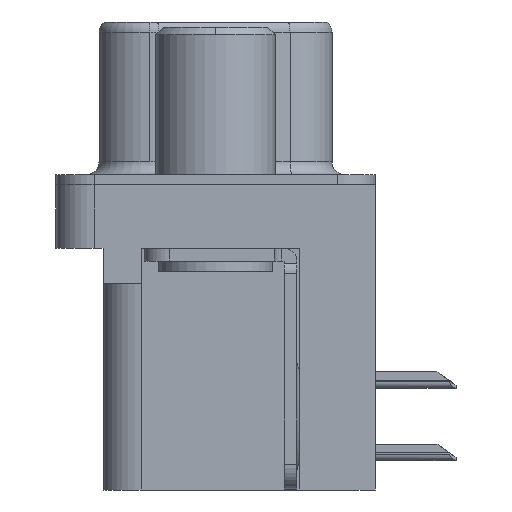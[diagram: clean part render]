
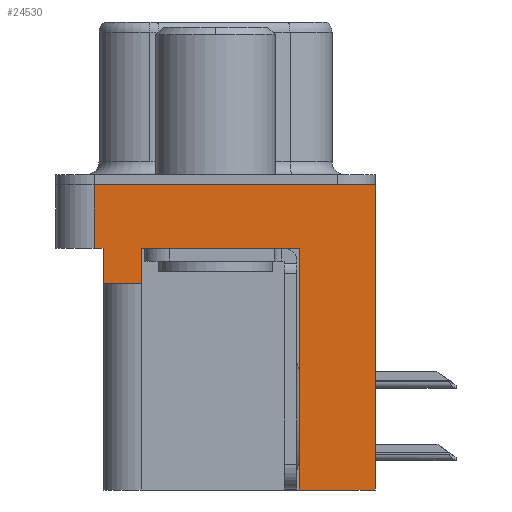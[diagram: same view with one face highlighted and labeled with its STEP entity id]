
A CAD part, left-side view. The second image highlights one B-rep face of the part: STEP entity #24530.
In plain terms, the highlighted planar face has unit normal (-1, 0, 0).
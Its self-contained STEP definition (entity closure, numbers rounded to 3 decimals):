
#223 = EDGE_CURVE ( 'NONE', #3522, #14569, #980, .T. ) ;
#358 = VECTOR ( 'NONE', #23700, 1000. ) ;
#980 = LINE ( 'NONE', #25428, #28120 ) ;
#1089 = EDGE_CURVE ( 'NONE', #8767, #10341, #22479, .T. ) ;
#1161 = CARTESIAN_POINT ( 'NONE',  ( -2.91, 2.895, -2.5 ) ) ;
#1478 = CARTESIAN_POINT ( 'NONE',  ( -2.91, -6.275, -2.5 ) ) ;
#2150 = VECTOR ( 'NONE', #5398, 1000. ) ;
#2228 = ORIENTED_EDGE ( 'NONE', *, *, #223, .T. ) ;
#2453 = CARTESIAN_POINT ( 'NONE',  ( -2.91, -6.275, -12. ) ) ;
#2769 = DIRECTION ( 'NONE',  ( 0., 0., 1. ) ) ;
#3426 = VERTEX_POINT ( 'NONE', #7520 ) ;
#3522 = VERTEX_POINT ( 'NONE', #1161 ) ;
#3541 = DIRECTION ( 'NONE',  ( 0., 0., 1. ) ) ;
#3948 = CARTESIAN_POINT ( 'NONE',  ( -2.91, 2.895, -3.9 ) ) ;
#4138 = ORIENTED_EDGE ( 'NONE', *, *, #10745, .F. ) ;
#4487 = EDGE_CURVE ( 'NONE', #10341, #17937, #27264, .T. ) ;
#4972 = LINE ( 'NONE', #16119, #2150 ) ;
#5138 = VECTOR ( 'NONE', #26257, 1000. ) ;
#5398 = DIRECTION ( 'NONE',  ( 0., 0., 1. ) ) ;
#5676 = ORIENTED_EDGE ( 'NONE', *, *, #19729, .F. ) ;
#5688 = VECTOR ( 'NONE', #17936, 1000. ) ;
#6105 = VECTOR ( 'NONE', #27433, 1000. ) ;
#6129 = CARTESIAN_POINT ( 'NONE',  ( -2.91, -3.295, -12. ) ) ;
#6491 = CARTESIAN_POINT ( 'NONE',  ( -2.91, -6.275, -2.5 ) ) ;
#6567 = ORIENTED_EDGE ( 'NONE', *, *, #21819, .F. ) ;
#6787 = DIRECTION ( 'NONE',  ( 0., -1., 0. ) ) ;
#7002 = LINE ( 'NONE', #1478, #358 ) ;
#7406 = LINE ( 'NONE', #27875, #10152 ) ;
#7520 = CARTESIAN_POINT ( 'NONE',  ( -2.91, 4.775, 0. ) ) ;
#8543 = EDGE_CURVE ( 'NONE', #8767, #3522, #23124, .T. ) ;
#8767 = VERTEX_POINT ( 'NONE', #3948 ) ;
#9052 = CARTESIAN_POINT ( 'NONE',  ( -2.91, -6.275, 0. ) ) ;
#9669 = DIRECTION ( 'NONE',  ( -1., 0., 0. ) ) ;
#10011 = DIRECTION ( 'NONE',  ( 0., 1., 0. ) ) ;
#10152 = VECTOR ( 'NONE', #10011, 1000. ) ;
#10341 = VERTEX_POINT ( 'NONE', #16968 ) ;
#10732 = ORIENTED_EDGE ( 'NONE', *, *, #15651, .T. ) ;
#10745 = EDGE_CURVE ( 'NONE', #25893, #14569, #28599, .T. ) ;
#11347 = ORIENTED_EDGE ( 'NONE', *, *, #4487, .F. ) ;
#13467 = VECTOR ( 'NONE', #6787, 1000. ) ;
#14061 = CARTESIAN_POINT ( 'NONE',  ( -2.91, -3.295, -12. ) ) ;
#14467 = VERTEX_POINT ( 'NONE', #15795 ) ;
#14569 = VERTEX_POINT ( 'NONE', #26089 ) ;
#14625 = CARTESIAN_POINT ( 'NONE',  ( -2.91, 2.895, -3.9 ) ) ;
#15651 = EDGE_CURVE ( 'NONE', #26917, #17937, #23138, .T. ) ;
#15701 = ORIENTED_EDGE ( 'NONE', *, *, #18604, .F. ) ;
#15795 = CARTESIAN_POINT ( 'NONE',  ( -2.91, -6.275, 0. ) ) ;
#16119 = CARTESIAN_POINT ( 'NONE',  ( -2.91, 4.775, -2.5 ) ) ;
#16616 = LINE ( 'NONE', #9052, #23511 ) ;
#16968 = CARTESIAN_POINT ( 'NONE',  ( -2.91, 4.425, -3.9 ) ) ;
#17782 = EDGE_LOOP ( 'NONE', ( #6567, #5676, #10732, #11347, #25589, #24689, #2228, #4138, #15701, #24806 ) ) ;
#17936 = DIRECTION ( 'NONE',  ( 0., 0., 1. ) ) ;
#17937 = VERTEX_POINT ( 'NONE', #21276 ) ;
#18543 = VERTEX_POINT ( 'NONE', #2453 ) ;
#18604 = EDGE_CURVE ( 'NONE', #18543, #25893, #7406, .T. ) ;
#18883 = CARTESIAN_POINT ( 'NONE',  ( -2.91, -6.275, -2.5 ) ) ;
#19236 = AXIS2_PLACEMENT_3D ( 'NONE', #18883, #9669, #3541 ) ;
#19729 = EDGE_CURVE ( 'NONE', #26917, #3426, #4972, .T. ) ;
#20173 = DIRECTION ( 'NONE',  ( 0., -1., 0. ) ) ;
#20711 = PLANE ( 'NONE',  #19236 ) ;
#21276 = CARTESIAN_POINT ( 'NONE',  ( -2.91, 4.425, -2.5 ) ) ;
#21819 = EDGE_CURVE ( 'NONE', #3426, #14467, #16616, .T. ) ;
#22479 = LINE ( 'NONE', #26452, #5138 ) ;
#22664 = FACE_OUTER_BOUND ( 'NONE', #17782, .T. ) ;
#22674 = VECTOR ( 'NONE', #2769, 1000. ) ;
#22870 = DIRECTION ( 'NONE',  ( 0., -1., 0. ) ) ;
#23124 = LINE ( 'NONE', #14625, #6105 ) ;
#23138 = LINE ( 'NONE', #6491, #13467 ) ;
#23511 = VECTOR ( 'NONE', #20173, 1000. ) ;
#23700 = DIRECTION ( 'NONE',  ( 0., 0., 1. ) ) ;
#23770 = CARTESIAN_POINT ( 'NONE',  ( -2.91, 4.775, -2.5 ) ) ;
#24530 = ADVANCED_FACE ( 'NONE', ( #22664 ), #20711, .T. ) ;
#24689 = ORIENTED_EDGE ( 'NONE', *, *, #8543, .T. ) ;
#24806 = ORIENTED_EDGE ( 'NONE', *, *, #26128, .T. ) ;
#25428 = CARTESIAN_POINT ( 'NONE',  ( -2.91, -6.275, -2.5 ) ) ;
#25589 = ORIENTED_EDGE ( 'NONE', *, *, #1089, .F. ) ;
#25893 = VERTEX_POINT ( 'NONE', #14061 ) ;
#26089 = CARTESIAN_POINT ( 'NONE',  ( -2.91, -3.295, -2.5 ) ) ;
#26128 = EDGE_CURVE ( 'NONE', #18543, #14467, #7002, .T. ) ;
#26257 = DIRECTION ( 'NONE',  ( 0., 1., 0. ) ) ;
#26452 = CARTESIAN_POINT ( 'NONE',  ( -2.91, 4.425, -3.9 ) ) ;
#26917 = VERTEX_POINT ( 'NONE', #23770 ) ;
#27264 = LINE ( 'NONE', #28797, #5688 ) ;
#27433 = DIRECTION ( 'NONE',  ( 0., 0., 1. ) ) ;
#27875 = CARTESIAN_POINT ( 'NONE',  ( -2.91, -3.295, -12. ) ) ;
#28120 = VECTOR ( 'NONE', #22870, 1000. ) ;
#28599 = LINE ( 'NONE', #6129, #22674 ) ;
#28797 = CARTESIAN_POINT ( 'NONE',  ( -2.91, 4.425, -3.9 ) ) ;
